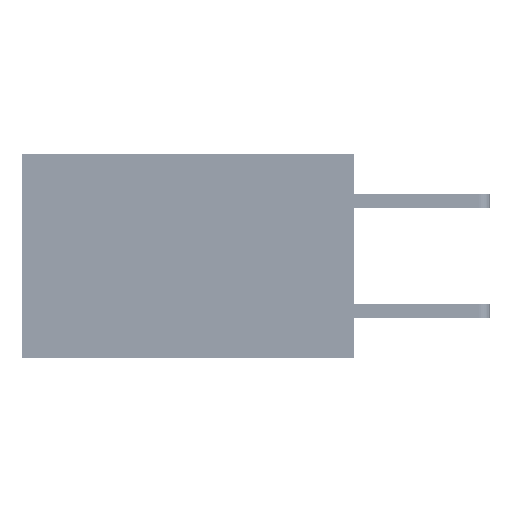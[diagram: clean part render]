
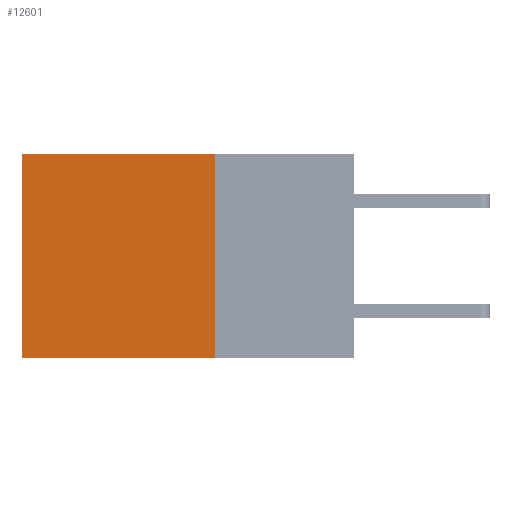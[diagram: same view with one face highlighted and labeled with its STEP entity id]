
A CAD part, left-side view. The second image highlights one B-rep face of the part: STEP entity #12601.
In plain terms, the highlighted planar face has unit normal (-1, 0, 0).
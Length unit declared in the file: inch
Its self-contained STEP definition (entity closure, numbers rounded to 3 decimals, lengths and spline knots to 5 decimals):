
#648 = DIRECTION ( 'NONE',  ( 0., 0., -1. ) ) ;
#786 = VECTOR ( 'NONE', #31936, 39.37008 ) ;
#3666 = LINE ( 'NONE', #21234, #28152 ) ;
#3835 = DIRECTION ( 'NONE',  ( 1., 0., 0. ) ) ;
#6391 = CARTESIAN_POINT ( 'NONE',  ( 0.2875, 0.6, -0.37 ) ) ;
#7170 = CARTESIAN_POINT ( 'NONE',  ( 0.2875, 0.25, 0. ) ) ;
#7371 = LINE ( 'NONE', #28270, #18889 ) ;
#7720 = LINE ( 'NONE', #34879, #786 ) ;
#9025 = ORIENTED_EDGE ( 'NONE', *, *, #31186, .T. ) ;
#10134 = VERTEX_POINT ( 'NONE', #6391 ) ;
#10632 = EDGE_CURVE ( 'NONE', #32385, #10134, #7371, .T. ) ;
#11183 = FACE_OUTER_BOUND ( 'NONE', #33462, .T. ) ;
#11713 = VECTOR ( 'NONE', #15070, 39.37008 ) ;
#12245 = LINE ( 'NONE', #34690, #11713 ) ;
#12361 = EDGE_CURVE ( 'NONE', #38446, #10134, #12245, .T. ) ;
#12601 = ADVANCED_FACE ( 'NONE', ( #11183 ), #39192, .F. ) ;
#13027 = EDGE_CURVE ( 'NONE', #14270, #38446, #3666, .T. ) ;
#14270 = VERTEX_POINT ( 'NONE', #15078 ) ;
#15070 = DIRECTION ( 'NONE',  ( 0., 1., 0. ) ) ;
#15078 = CARTESIAN_POINT ( 'NONE',  ( 0.2875, 0.25, 0. ) ) ;
#15248 = ORIENTED_EDGE ( 'NONE', *, *, #10632, .T. ) ;
#16109 = ORIENTED_EDGE ( 'NONE', *, *, #12361, .F. ) ;
#17546 = CARTESIAN_POINT ( 'NONE',  ( 0.2875, 0.25, -0.37 ) ) ;
#18889 = VECTOR ( 'NONE', #31328, 39.37008 ) ;
#21234 = CARTESIAN_POINT ( 'NONE',  ( 0.2875, 0.25, 0. ) ) ;
#27687 = CARTESIAN_POINT ( 'NONE',  ( 0.2875, 0.6, 0. ) ) ;
#28152 = VECTOR ( 'NONE', #35338, 39.37008 ) ;
#28270 = CARTESIAN_POINT ( 'NONE',  ( 0.2875, 0.6, 0. ) ) ;
#31186 = EDGE_CURVE ( 'NONE', #14270, #32385, #7720, .T. ) ;
#31328 = DIRECTION ( 'NONE',  ( 0., 0., -1. ) ) ;
#31936 = DIRECTION ( 'NONE',  ( 0., 1., 0. ) ) ;
#32385 = VERTEX_POINT ( 'NONE', #27687 ) ;
#33462 = EDGE_LOOP ( 'NONE', ( #15248, #16109, #38592, #9025 ) ) ;
#34690 = CARTESIAN_POINT ( 'NONE',  ( 0.2875, 0.25, -0.37 ) ) ;
#34879 = CARTESIAN_POINT ( 'NONE',  ( 0.2875, 0.25, 0. ) ) ;
#35338 = DIRECTION ( 'NONE',  ( 0., 0., -1. ) ) ;
#38446 = VERTEX_POINT ( 'NONE', #17546 ) ;
#38592 = ORIENTED_EDGE ( 'NONE', *, *, #13027, .F. ) ;
#39164 = AXIS2_PLACEMENT_3D ( 'NONE', #7170, #3835, #648 ) ;
#39192 = PLANE ( 'NONE',  #39164 ) ;
